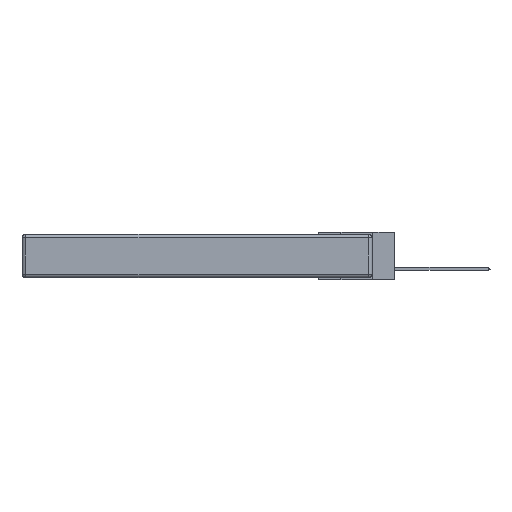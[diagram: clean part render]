
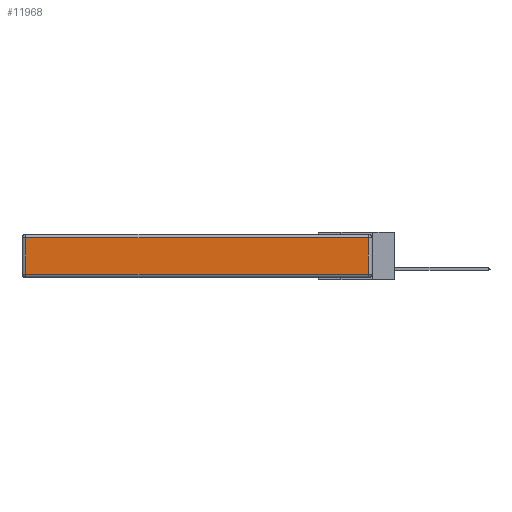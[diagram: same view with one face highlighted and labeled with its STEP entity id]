
A CAD part, left-side view. The second image highlights one B-rep face of the part: STEP entity #11968.
In plain terms, the highlighted planar face has unit normal (-1, 0, 0).
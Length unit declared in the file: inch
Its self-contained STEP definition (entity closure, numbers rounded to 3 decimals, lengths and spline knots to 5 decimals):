
#878 = DIRECTION ( 'NONE',  ( 0., 0., 1. ) ) ;
#1075 = ORIENTED_EDGE ( 'NONE', *, *, #24515, .T. ) ;
#1272 = LINE ( 'NONE', #2910, #26933 ) ;
#2910 = CARTESIAN_POINT ( 'NONE',  ( 0., 2.75, -0.03 ) ) ;
#3740 = AXIS2_PLACEMENT_3D ( 'NONE', #16746, #6075, #878 ) ;
#4638 = VECTOR ( 'NONE', #22669, 39.37008 ) ;
#6075 = DIRECTION ( 'NONE',  ( -1., 0., 0. ) ) ;
#6806 = CARTESIAN_POINT ( 'NONE',  ( 0., 2.72, -0.343 ) ) ;
#7267 = VERTEX_POINT ( 'NONE', #22117 ) ;
#10700 = DIRECTION ( 'NONE',  ( 0., 1., 0. ) ) ;
#10886 = LINE ( 'NONE', #17236, #4638 ) ;
#11741 = DIRECTION ( 'NONE',  ( 0., -1., 0. ) ) ;
#11968 = ADVANCED_FACE ( 'NONE', ( #14985 ), #21723, .T. ) ;
#12209 = EDGE_CURVE ( 'NONE', #29132, #7267, #1272, .T. ) ;
#12377 = ORIENTED_EDGE ( 'NONE', *, *, #12209, .T. ) ;
#14985 = FACE_OUTER_BOUND ( 'NONE', #30174, .T. ) ;
#16176 = VERTEX_POINT ( 'NONE', #26175 ) ;
#16278 = LINE ( 'NONE', #19927, #26621 ) ;
#16746 = CARTESIAN_POINT ( 'NONE',  ( 0., 0., -0.343 ) ) ;
#16957 = VERTEX_POINT ( 'NONE', #17773 ) ;
#17236 = CARTESIAN_POINT ( 'NONE',  ( 0., 0.03, -0.343 ) ) ;
#17773 = CARTESIAN_POINT ( 'NONE',  ( 0., 0.03, -0.313 ) ) ;
#18245 = CARTESIAN_POINT ( 'NONE',  ( 0., 0.03, -0.03 ) ) ;
#19835 = EDGE_CURVE ( 'NONE', #7267, #16176, #20079, .T. ) ;
#19927 = CARTESIAN_POINT ( 'NONE',  ( 0., 0., -0.313 ) ) ;
#20079 = LINE ( 'NONE', #6806, #26267 ) ;
#21723 = PLANE ( 'NONE',  #3740 ) ;
#22117 = CARTESIAN_POINT ( 'NONE',  ( 0., 2.72, -0.03 ) ) ;
#22669 = DIRECTION ( 'NONE',  ( 0., 0., 1. ) ) ;
#23898 = ORIENTED_EDGE ( 'NONE', *, *, #19835, .T. ) ;
#24197 = EDGE_CURVE ( 'NONE', #16176, #16957, #16278, .T. ) ;
#24515 = EDGE_CURVE ( 'NONE', #16957, #29132, #10886, .T. ) ;
#26175 = CARTESIAN_POINT ( 'NONE',  ( 0., 2.72, -0.313 ) ) ;
#26267 = VECTOR ( 'NONE', #28103, 39.37008 ) ;
#26621 = VECTOR ( 'NONE', #11741, 39.37008 ) ;
#26933 = VECTOR ( 'NONE', #10700, 39.37008 ) ;
#28103 = DIRECTION ( 'NONE',  ( 0., 0., -1. ) ) ;
#29132 = VERTEX_POINT ( 'NONE', #18245 ) ;
#30174 = EDGE_LOOP ( 'NONE', ( #30875, #1075, #12377, #23898 ) ) ;
#30875 = ORIENTED_EDGE ( 'NONE', *, *, #24197, .T. ) ;
